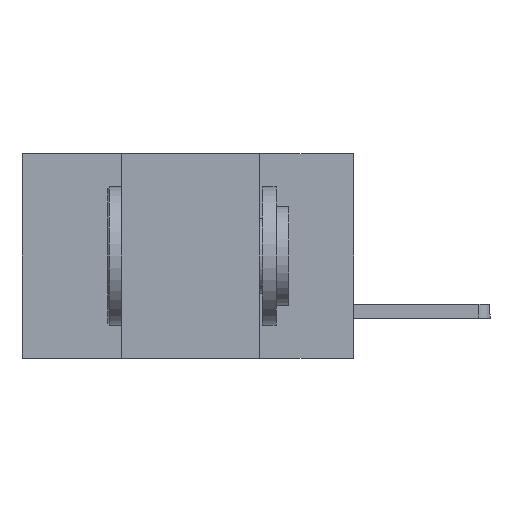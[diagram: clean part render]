
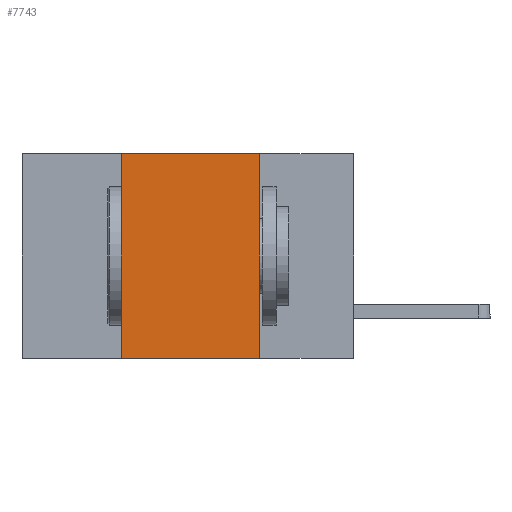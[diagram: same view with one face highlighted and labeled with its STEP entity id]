
A CAD part, left-side view. The second image highlights one B-rep face of the part: STEP entity #7743.
In plain terms, the highlighted planar face has unit normal (-1, 0, 0).
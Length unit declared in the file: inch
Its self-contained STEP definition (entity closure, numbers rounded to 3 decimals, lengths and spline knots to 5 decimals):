
#202 = PLANE ( 'NONE',  #5068 ) ;
#262 = ORIENTED_EDGE ( 'NONE', *, *, #6685, .F. ) ;
#330 = ORIENTED_EDGE ( 'NONE', *, *, #8906, .F. ) ;
#334 = ORIENTED_EDGE ( 'NONE', *, *, #9624, .F. ) ;
#378 = ORIENTED_EDGE ( 'NONE', *, *, #7808, .T. ) ;
#1058 = VERTEX_POINT ( 'NONE', #6788 ) ;
#1199 = VERTEX_POINT ( 'NONE', #8579 ) ;
#1280 = DIRECTION ( 'NONE',  ( 0., -1., 0. ) ) ;
#1455 = CARTESIAN_POINT ( 'NONE',  ( 0., 0.42, 0. ) ) ;
#2281 = DIRECTION ( 'NONE',  ( 0., -1., 0. ) ) ;
#2372 = DIRECTION ( 'NONE',  ( 0., 0., 1. ) ) ;
#2468 = LINE ( 'NONE', #6755, #11038 ) ;
#2864 = CARTESIAN_POINT ( 'NONE',  ( 0., 0.42, 0. ) ) ;
#2924 = VECTOR ( 'NONE', #1280, 39.37008 ) ;
#3214 = LINE ( 'NONE', #5817, #2924 ) ;
#3800 = FACE_OUTER_BOUND ( 'NONE', #9312, .T. ) ;
#3889 = VECTOR ( 'NONE', #2372, 39.37008 ) ;
#4157 = LINE ( 'NONE', #1455, #3889 ) ;
#5068 = AXIS2_PLACEMENT_3D ( 'NONE', #9952, #10750, #5740 ) ;
#5740 = DIRECTION ( 'NONE',  ( 0., 0., -1. ) ) ;
#5817 = CARTESIAN_POINT ( 'NONE',  ( 0., 0.6, -0.37 ) ) ;
#5928 = DIRECTION ( 'NONE',  ( 0., 0., -1. ) ) ;
#6049 = VECTOR ( 'NONE', #5928, 39.37008 ) ;
#6401 = VERTEX_POINT ( 'NONE', #2864 ) ;
#6685 = EDGE_CURVE ( 'NONE', #1199, #1058, #8300, .T. ) ;
#6755 = CARTESIAN_POINT ( 'NONE',  ( 0., 0.6, 0. ) ) ;
#6788 = CARTESIAN_POINT ( 'NONE',  ( 0., 0.17, -0.37 ) ) ;
#7743 = ADVANCED_FACE ( 'NONE', ( #3800 ), #202, .F. ) ;
#7808 = EDGE_CURVE ( 'NONE', #9218, #1058, #3214, .T. ) ;
#8300 = LINE ( 'NONE', #10142, #6049 ) ;
#8579 = CARTESIAN_POINT ( 'NONE',  ( 0., 0.17, 0. ) ) ;
#8906 = EDGE_CURVE ( 'NONE', #6401, #1199, #2468, .T. ) ;
#9218 = VERTEX_POINT ( 'NONE', #10423 ) ;
#9312 = EDGE_LOOP ( 'NONE', ( #262, #330, #334, #378 ) ) ;
#9624 = EDGE_CURVE ( 'NONE', #9218, #6401, #4157, .T. ) ;
#9952 = CARTESIAN_POINT ( 'NONE',  ( 0., 0.6, 0. ) ) ;
#10142 = CARTESIAN_POINT ( 'NONE',  ( 0., 0.17, 0. ) ) ;
#10423 = CARTESIAN_POINT ( 'NONE',  ( 0., 0.42, -0.37 ) ) ;
#10750 = DIRECTION ( 'NONE',  ( 1., 0., 0. ) ) ;
#11038 = VECTOR ( 'NONE', #2281, 39.37008 ) ;
